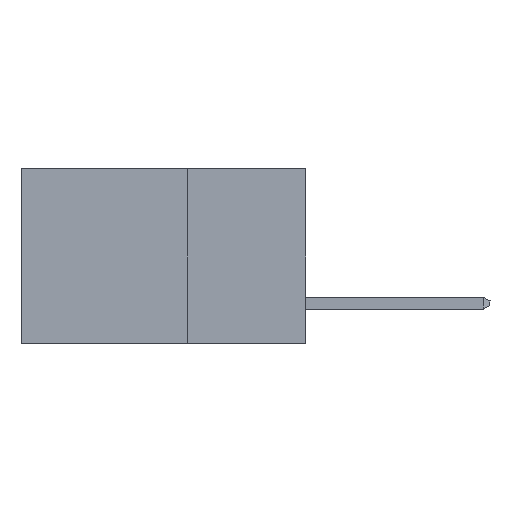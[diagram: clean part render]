
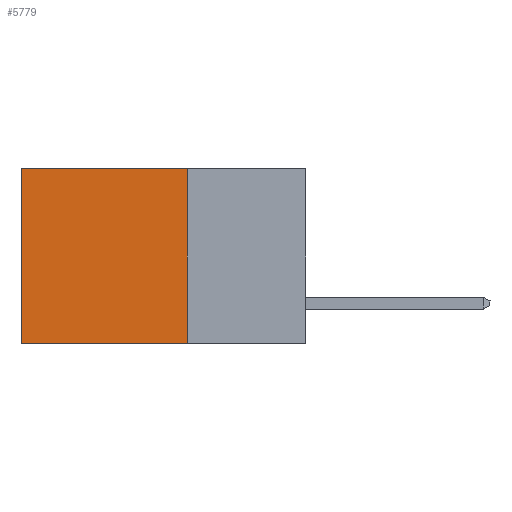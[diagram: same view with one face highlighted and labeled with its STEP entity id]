
A CAD part, left-side view. The second image highlights one B-rep face of the part: STEP entity #5779.
In plain terms, the highlighted planar face has unit normal (-1, 0, 0).
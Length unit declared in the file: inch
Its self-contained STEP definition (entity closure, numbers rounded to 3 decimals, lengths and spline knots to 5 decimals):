
#336 = CARTESIAN_POINT ( 'NONE',  ( 0.2615, 0.25, -0.37 ) ) ;
#525 = EDGE_CURVE ( 'NONE', #6846, #557, #6722, .T. ) ;
#557 = VERTEX_POINT ( 'NONE', #7937 ) ;
#1137 = EDGE_LOOP ( 'NONE', ( #5962, #7657, #4171, #7951 ) ) ;
#1390 = CARTESIAN_POINT ( 'NONE',  ( 0.2615, 0.25, -0.37 ) ) ;
#1756 = VECTOR ( 'NONE', #6505, 39.37008 ) ;
#2446 = LINE ( 'NONE', #5795, #4181 ) ;
#2553 = DIRECTION ( 'NONE',  ( 0., 1., 0. ) ) ;
#2726 = LINE ( 'NONE', #4313, #5882 ) ;
#3115 = EDGE_CURVE ( 'NONE', #557, #3862, #3165, .T. ) ;
#3165 = LINE ( 'NONE', #4037, #1756 ) ;
#3650 = VERTEX_POINT ( 'NONE', #336 ) ;
#3862 = VERTEX_POINT ( 'NONE', #8341 ) ;
#4006 = EDGE_CURVE ( 'NONE', #6846, #3650, #2726, .T. ) ;
#4037 = CARTESIAN_POINT ( 'NONE',  ( 0.2615, 0.6, -0.37 ) ) ;
#4171 = ORIENTED_EDGE ( 'NONE', *, *, #4006, .F. ) ;
#4181 = VECTOR ( 'NONE', #5843, 39.37008 ) ;
#4313 = CARTESIAN_POINT ( 'NONE',  ( 0.2615, 0.25, -0.37 ) ) ;
#4371 = DIRECTION ( 'NONE',  ( 0., 0., -1. ) ) ;
#5779 = ADVANCED_FACE ( 'NONE', ( #6336 ), #9619, .F. ) ;
#5795 = CARTESIAN_POINT ( 'NONE',  ( 0.2615, 0.25, -0.37 ) ) ;
#5843 = DIRECTION ( 'NONE',  ( 0., 1., 0. ) ) ;
#5882 = VECTOR ( 'NONE', #4371, 39.37008 ) ;
#5962 = ORIENTED_EDGE ( 'NONE', *, *, #3115, .T. ) ;
#6261 = AXIS2_PLACEMENT_3D ( 'NONE', #1390, #7083, #8927 ) ;
#6336 = FACE_OUTER_BOUND ( 'NONE', #1137, .T. ) ;
#6505 = DIRECTION ( 'NONE',  ( 0., 0., -1. ) ) ;
#6722 = LINE ( 'NONE', #6829, #6893 ) ;
#6829 = CARTESIAN_POINT ( 'NONE',  ( 0.2615, 0.25, 0. ) ) ;
#6846 = VERTEX_POINT ( 'NONE', #6929 ) ;
#6893 = VECTOR ( 'NONE', #2553, 39.37008 ) ;
#6929 = CARTESIAN_POINT ( 'NONE',  ( 0.2615, 0.25, 0. ) ) ;
#7083 = DIRECTION ( 'NONE',  ( 1., 0., 0. ) ) ;
#7657 = ORIENTED_EDGE ( 'NONE', *, *, #8320, .F. ) ;
#7937 = CARTESIAN_POINT ( 'NONE',  ( 0.2615, 0.6, 0. ) ) ;
#7951 = ORIENTED_EDGE ( 'NONE', *, *, #525, .T. ) ;
#8320 = EDGE_CURVE ( 'NONE', #3650, #3862, #2446, .T. ) ;
#8341 = CARTESIAN_POINT ( 'NONE',  ( 0.2615, 0.6, -0.37 ) ) ;
#8927 = DIRECTION ( 'NONE',  ( 0., 0., -1. ) ) ;
#9619 = PLANE ( 'NONE',  #6261 ) ;
